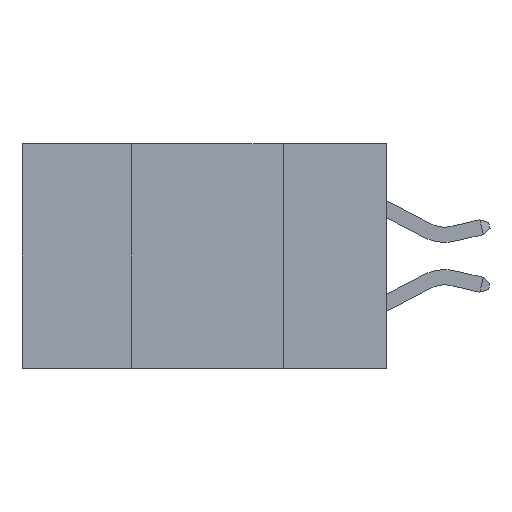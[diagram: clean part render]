
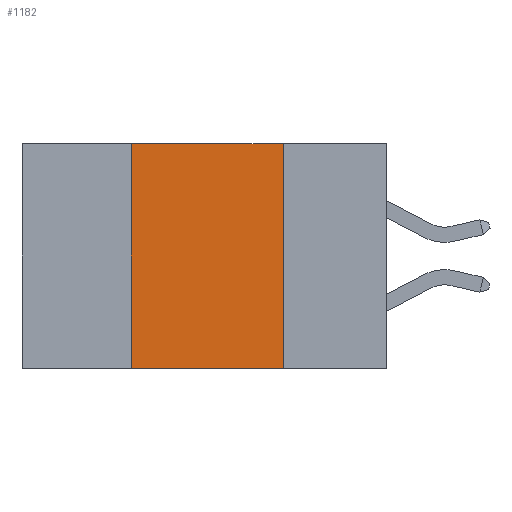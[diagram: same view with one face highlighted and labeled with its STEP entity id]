
A CAD part, left-side view. The second image highlights one B-rep face of the part: STEP entity #1182.
In plain terms, the highlighted planar face has unit normal (-1, 0, 0).
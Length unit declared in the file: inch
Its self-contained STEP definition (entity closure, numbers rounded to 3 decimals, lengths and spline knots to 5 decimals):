
#110 = CARTESIAN_POINT ( 'NONE',  ( 0., 0.6, -0.37 ) ) ;
#126 = EDGE_CURVE ( 'NONE', #5974, #983, #9992, .T. ) ;
#530 = CARTESIAN_POINT ( 'NONE',  ( 0., 0.42, 0. ) ) ;
#665 = AXIS2_PLACEMENT_3D ( 'NONE', #9789, #7819, #6567 ) ;
#819 = ORIENTED_EDGE ( 'NONE', *, *, #3360, .T. ) ;
#983 = VERTEX_POINT ( 'NONE', #530 ) ;
#1182 = ADVANCED_FACE ( 'NONE', ( #8173 ), #4906, .F. ) ;
#1243 = LINE ( 'NONE', #3206, #6232 ) ;
#1515 = EDGE_CURVE ( 'NONE', #5695, #2045, #1243, .T. ) ;
#1838 = LINE ( 'NONE', #110, #6526 ) ;
#2045 = VERTEX_POINT ( 'NONE', #8338 ) ;
#2865 = ORIENTED_EDGE ( 'NONE', *, *, #11052, .F. ) ;
#3206 = CARTESIAN_POINT ( 'NONE',  ( 0., 0.17, 0. ) ) ;
#3360 = EDGE_CURVE ( 'NONE', #5974, #2045, #1838, .T. ) ;
#4104 = DIRECTION ( 'NONE',  ( 0., -1., 0. ) ) ;
#4512 = DIRECTION ( 'NONE',  ( 0., 0., 1. ) ) ;
#4706 = EDGE_LOOP ( 'NONE', ( #9102, #2865, #11690, #819 ) ) ;
#4906 = PLANE ( 'NONE',  #665 ) ;
#5695 = VERTEX_POINT ( 'NONE', #7418 ) ;
#5974 = VERTEX_POINT ( 'NONE', #9757 ) ;
#6232 = VECTOR ( 'NONE', #7756, 39.37008 ) ;
#6526 = VECTOR ( 'NONE', #11429, 39.37008 ) ;
#6567 = DIRECTION ( 'NONE',  ( 0., 0., -1. ) ) ;
#7308 = VECTOR ( 'NONE', #4104, 39.37008 ) ;
#7418 = CARTESIAN_POINT ( 'NONE',  ( 0., 0.17, 0. ) ) ;
#7470 = VECTOR ( 'NONE', #4512, 39.37008 ) ;
#7756 = DIRECTION ( 'NONE',  ( 0., 0., -1. ) ) ;
#7819 = DIRECTION ( 'NONE',  ( 1., 0., 0. ) ) ;
#8173 = FACE_OUTER_BOUND ( 'NONE', #4706, .T. ) ;
#8338 = CARTESIAN_POINT ( 'NONE',  ( 0., 0.17, -0.37 ) ) ;
#9102 = ORIENTED_EDGE ( 'NONE', *, *, #1515, .F. ) ;
#9757 = CARTESIAN_POINT ( 'NONE',  ( 0., 0.42, -0.37 ) ) ;
#9789 = CARTESIAN_POINT ( 'NONE',  ( 0., 0.6, 0. ) ) ;
#9810 = LINE ( 'NONE', #11611, #7308 ) ;
#9992 = LINE ( 'NONE', #11600, #7470 ) ;
#11052 = EDGE_CURVE ( 'NONE', #983, #5695, #9810, .T. ) ;
#11429 = DIRECTION ( 'NONE',  ( 0., -1., 0. ) ) ;
#11600 = CARTESIAN_POINT ( 'NONE',  ( 0., 0.42, 0. ) ) ;
#11611 = CARTESIAN_POINT ( 'NONE',  ( 0., 0.6, 0. ) ) ;
#11690 = ORIENTED_EDGE ( 'NONE', *, *, #126, .F. ) ;
